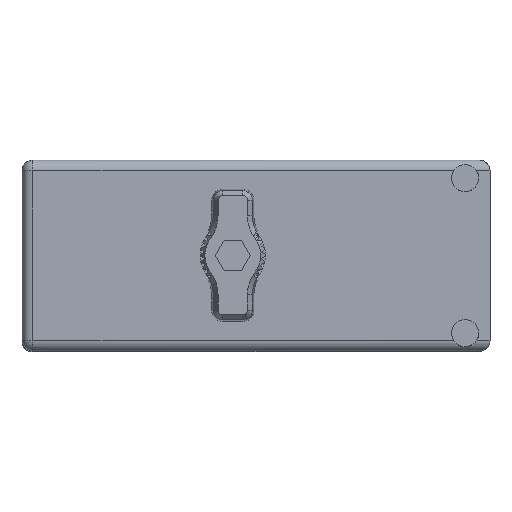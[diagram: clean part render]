
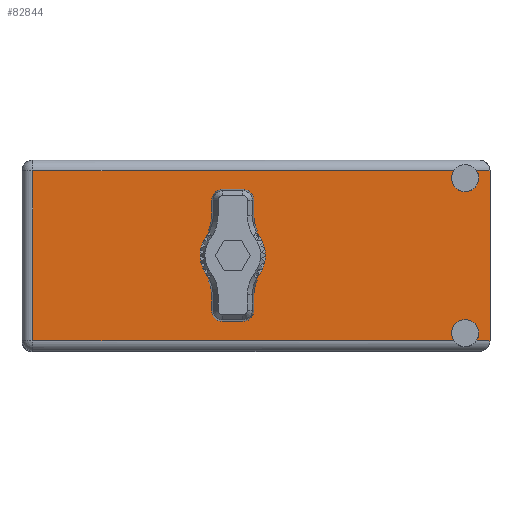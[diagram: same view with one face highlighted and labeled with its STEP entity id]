
A CAD part, top view. The second image highlights one B-rep face of the part: STEP entity #82844.
In plain terms, the highlighted face is planar.
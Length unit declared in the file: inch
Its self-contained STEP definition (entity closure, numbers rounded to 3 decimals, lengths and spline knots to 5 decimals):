
#594 = AXIS2_PLACEMENT_3D ( 'NONE', #15617, #9534, #87026 ) ;
#677 = DIRECTION ( 'NONE',  ( 0., 0., 1. ) ) ;
#2034 = VERTEX_POINT ( 'NONE', #17839 ) ;
#4506 = DIRECTION ( 'NONE',  ( 1., 0., 0. ) ) ;
#4629 = ORIENTED_EDGE ( 'NONE', *, *, #35222, .T. ) ;
#4676 = EDGE_CURVE ( 'NONE', #75758, #20215, #31392, .T. ) ;
#5254 = LINE ( 'NONE', #67888, #21703 ) ;
#6256 = DIRECTION ( 'NONE',  ( 0., 1., 0. ) ) ;
#6964 = ORIENTED_EDGE ( 'NONE', *, *, #9692, .F. ) ;
#7058 = DIRECTION ( 'NONE',  ( 0., 0., 1. ) ) ;
#9191 = CARTESIAN_POINT ( 'NONE',  ( 1.499, 1.675, -0.5 ) ) ;
#9534 = DIRECTION ( 'NONE',  ( 0., 1., 0. ) ) ;
#9692 = EDGE_CURVE ( 'NONE', #54153, #20215, #58096, .T. ) ;
#10877 = CIRCLE ( 'NONE', #26780, 0.125 ) ;
#11030 = CARTESIAN_POINT ( 'NONE',  ( 1.42519, 1.675, -0.547 ) ) ;
#11601 = CARTESIAN_POINT ( 'NONE',  ( 1.499, 1.675, 0.5 ) ) ;
#11673 = LINE ( 'NONE', #49350, #73370 ) ;
#12789 = DIRECTION ( 'NONE',  ( 0., 1., 0. ) ) ;
#12853 = ORIENTED_EDGE ( 'NONE', *, *, #35820, .F. ) ;
#13084 = VERTEX_POINT ( 'NONE', #50749 ) ;
#13308 = CARTESIAN_POINT ( 'NONE',  ( 1.499, 1.675, -0.5 ) ) ;
#14794 = EDGE_CURVE ( 'NONE', #13084, #45931, #74985, .T. ) ;
#15334 = AXIS2_PLACEMENT_3D ( 'NONE', #26908, #6256, #677 ) ;
#15617 = CARTESIAN_POINT ( 'NONE',  ( -1.359, 1.675, -0.617 ) ) ;
#17839 = CARTESIAN_POINT ( 'NONE',  ( 1.42519, 1.675, 0.547 ) ) ;
#17875 = DIRECTION ( 'NONE',  ( 1., 0., 0. ) ) ;
#20215 = VERTEX_POINT ( 'NONE', #37892 ) ;
#21529 = VERTEX_POINT ( 'NONE', #11030 ) ;
#21703 = VECTOR ( 'NONE', #61136, 39.37008 ) ;
#21959 = VECTOR ( 'NONE', #17875, 39.37008 ) ;
#22612 = CIRCLE ( 'NONE', #56769, 0.0875 ) ;
#23220 = EDGE_CURVE ( 'NONE', #54145, #42921, #84006, .T. ) ;
#23334 = DIRECTION ( 'NONE',  ( 0., 0., 1. ) ) ;
#23708 = VECTOR ( 'NONE', #47399, 39.37008 ) ;
#24045 = VECTOR ( 'NONE', #28717, 39.37008 ) ;
#25874 = CARTESIAN_POINT ( 'NONE',  ( -1.359, 1.675, -0.547 ) ) ;
#26780 = AXIS2_PLACEMENT_3D ( 'NONE', #49505, #84509, #7058 ) ;
#26908 = CARTESIAN_POINT ( 'NONE',  ( 0., 1.675, 0. ) ) ;
#27373 = VERTEX_POINT ( 'NONE', #64121 ) ;
#27791 = CARTESIAN_POINT ( 'NONE',  ( 0., 1.675, -0.125 ) ) ;
#28717 = DIRECTION ( 'NONE',  ( 0., 0., 1. ) ) ;
#29071 = EDGE_CURVE ( 'NONE', #57510, #2034, #50285, .T. ) ;
#31392 = LINE ( 'NONE', #25874, #23708 ) ;
#32101 = CIRCLE ( 'NONE', #52912, 0.0875 ) ;
#34375 = ORIENTED_EDGE ( 'NONE', *, *, #77010, .F. ) ;
#35222 = EDGE_CURVE ( 'NONE', #59609, #27373, #11673, .T. ) ;
#35820 = EDGE_CURVE ( 'NONE', #13084, #57510, #22612, .T. ) ;
#37064 = CARTESIAN_POINT ( 'NONE',  ( -1.289, 1.675, -0.547 ) ) ;
#37817 = CARTESIAN_POINT ( 'NONE',  ( 1.499, 1.675, 0.5 ) ) ;
#37892 = CARTESIAN_POINT ( 'NONE',  ( 1.57281, 1.675, -0.547 ) ) ;
#39271 = ORIENTED_EDGE ( 'NONE', *, *, #55553, .F. ) ;
#39488 = EDGE_CURVE ( 'NONE', #21529, #54153, #32101, .T. ) ;
#40219 = DIRECTION ( 'NONE',  ( 0., 0., 1. ) ) ;
#42921 = VERTEX_POINT ( 'NONE', #27791 ) ;
#42968 = AXIS2_PLACEMENT_3D ( 'NONE', #11601, #12789, #40219 ) ;
#43500 = CARTESIAN_POINT ( 'NONE',  ( 1.659, 1.675, 0.617 ) ) ;
#43700 = CARTESIAN_POINT ( 'NONE',  ( 1.499, 1.675, -0.4125 ) ) ;
#44062 = LINE ( 'NONE', #53002, #21959 ) ;
#45370 = VECTOR ( 'NONE', #4506, 39.37008 ) ;
#45931 = VERTEX_POINT ( 'NONE', #60518 ) ;
#46767 = EDGE_CURVE ( 'NONE', #21529, #59609, #5254, .T. ) ;
#47399 = DIRECTION ( 'NONE',  ( -1., 0., 0. ) ) ;
#49350 = CARTESIAN_POINT ( 'NONE',  ( -1.289, 1.675, -0.617 ) ) ;
#49505 = CARTESIAN_POINT ( 'NONE',  ( 0., 1.675, 0. ) ) ;
#50285 = CIRCLE ( 'NONE', #42968, 0.0875 ) ;
#50462 = ORIENTED_EDGE ( 'NONE', *, *, #52916, .T. ) ;
#50749 = CARTESIAN_POINT ( 'NONE',  ( 1.57281, 1.675, 0.547 ) ) ;
#52912 = AXIS2_PLACEMENT_3D ( 'NONE', #9191, #79606, #23334 ) ;
#52916 = EDGE_CURVE ( 'NONE', #27373, #2034, #44062, .T. ) ;
#53002 = CARTESIAN_POINT ( 'NONE',  ( 1.659, 1.675, 0.547 ) ) ;
#54145 = VERTEX_POINT ( 'NONE', #57799 ) ;
#54153 = VERTEX_POINT ( 'NONE', #43700 ) ;
#55514 = CARTESIAN_POINT ( 'NONE',  ( 1.499, 1.675, 0.4125 ) ) ;
#55553 = EDGE_CURVE ( 'NONE', #42921, #54145, #10877, .T. ) ;
#56769 = AXIS2_PLACEMENT_3D ( 'NONE', #37817, #86383, #79632 ) ;
#57510 = VERTEX_POINT ( 'NONE', #55514 ) ;
#57799 = CARTESIAN_POINT ( 'NONE',  ( 0., 1.675, 0.125 ) ) ;
#58096 = CIRCLE ( 'NONE', #76695, 0.0875 ) ;
#58432 = PLANE ( 'NONE',  #594 ) ;
#59609 = VERTEX_POINT ( 'NONE', #37064 ) ;
#60518 = CARTESIAN_POINT ( 'NONE',  ( 1.659, 1.675, 0.547 ) ) ;
#60626 = CARTESIAN_POINT ( 'NONE',  ( 1.659, 1.675, -0.547 ) ) ;
#61136 = DIRECTION ( 'NONE',  ( -1., 0., 0. ) ) ;
#61401 = DIRECTION ( 'NONE',  ( 0., 0., 1. ) ) ;
#64121 = CARTESIAN_POINT ( 'NONE',  ( -1.289, 1.675, 0.547 ) ) ;
#66209 = ORIENTED_EDGE ( 'NONE', *, *, #14794, .T. ) ;
#67535 = CARTESIAN_POINT ( 'NONE',  ( 1.659, 1.675, 0.547 ) ) ;
#67764 = ORIENTED_EDGE ( 'NONE', *, *, #46767, .T. ) ;
#67888 = CARTESIAN_POINT ( 'NONE',  ( -1.359, 1.675, -0.547 ) ) ;
#70390 = EDGE_LOOP ( 'NONE', ( #50462, #77554, #12853, #66209, #34375, #71167, #6964, #88508, #67764, #4629 ) ) ;
#71167 = ORIENTED_EDGE ( 'NONE', *, *, #4676, .T. ) ;
#73370 = VECTOR ( 'NONE', #77614, 39.37008 ) ;
#73770 = FACE_BOUND ( 'NONE', #85333, .T. ) ;
#74985 = LINE ( 'NONE', #67535, #45370 ) ;
#75732 = LINE ( 'NONE', #43500, #24045 ) ;
#75758 = VERTEX_POINT ( 'NONE', #60626 ) ;
#76695 = AXIS2_PLACEMENT_3D ( 'NONE', #13308, #89656, #61401 ) ;
#77010 = EDGE_CURVE ( 'NONE', #75758, #45931, #75732, .T. ) ;
#77554 = ORIENTED_EDGE ( 'NONE', *, *, #29071, .F. ) ;
#77614 = DIRECTION ( 'NONE',  ( 0., 0., 1. ) ) ;
#77987 = ORIENTED_EDGE ( 'NONE', *, *, #23220, .F. ) ;
#79606 = DIRECTION ( 'NONE',  ( 0., 1., 0. ) ) ;
#79632 = DIRECTION ( 'NONE',  ( 0., 0., 1. ) ) ;
#80405 = FACE_OUTER_BOUND ( 'NONE', #70390, .T. ) ;
#82844 = ADVANCED_FACE ( 'NONE', ( #73770, #80405 ), #58432, .T. ) ;
#84006 = CIRCLE ( 'NONE', #15334, 0.125 ) ;
#84509 = DIRECTION ( 'NONE',  ( 0., 1., 0. ) ) ;
#85333 = EDGE_LOOP ( 'NONE', ( #77987, #39271 ) ) ;
#86383 = DIRECTION ( 'NONE',  ( 0., 1., 0. ) ) ;
#87026 = DIRECTION ( 'NONE',  ( -1., 0., 0. ) ) ;
#88508 = ORIENTED_EDGE ( 'NONE', *, *, #39488, .F. ) ;
#89656 = DIRECTION ( 'NONE',  ( 0., 1., 0. ) ) ;
